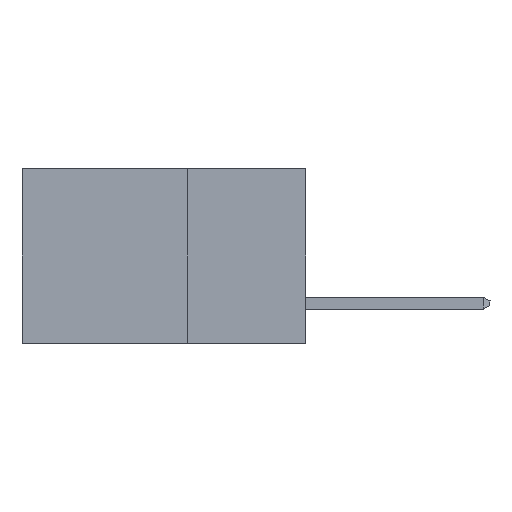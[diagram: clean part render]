
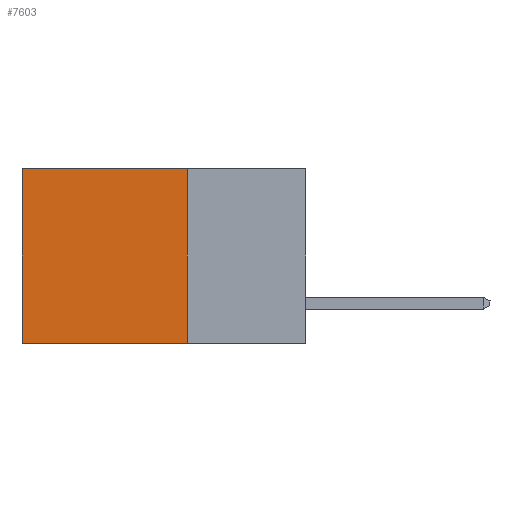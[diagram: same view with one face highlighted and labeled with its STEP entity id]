
A CAD part, left-side view. The second image highlights one B-rep face of the part: STEP entity #7603.
In plain terms, the highlighted planar face has unit normal (-1, 0, 0).
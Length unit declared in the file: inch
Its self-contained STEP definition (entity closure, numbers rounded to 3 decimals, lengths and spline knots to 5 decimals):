
#1020 = VERTEX_POINT ( 'NONE', #2128 ) ;
#2128 = CARTESIAN_POINT ( 'NONE',  ( 0.298, 0.25, -0.37 ) ) ;
#2580 = EDGE_LOOP ( 'NONE', ( #7475, #16033, #7656, #6407 ) ) ;
#3238 = LINE ( 'NONE', #11141, #9795 ) ;
#3564 = DIRECTION ( 'NONE',  ( 0., 1., 0. ) ) ;
#3631 = LINE ( 'NONE', #15164, #6286 ) ;
#3902 = AXIS2_PLACEMENT_3D ( 'NONE', #6170, #16799, #8783 ) ;
#5137 = VECTOR ( 'NONE', #12179, 39.37008 ) ;
#5731 = EDGE_CURVE ( 'NONE', #11971, #14548, #3631, .T. ) ;
#6170 = CARTESIAN_POINT ( 'NONE',  ( 0.298, 0.25, 0. ) ) ;
#6286 = VECTOR ( 'NONE', #11231, 39.37008 ) ;
#6407 = ORIENTED_EDGE ( 'NONE', *, *, #7069, .T. ) ;
#7069 = EDGE_CURVE ( 'NONE', #8485, #11971, #15733, .T. ) ;
#7475 = ORIENTED_EDGE ( 'NONE', *, *, #5731, .T. ) ;
#7603 = ADVANCED_FACE ( 'NONE', ( #16939 ), #15314, .F. ) ;
#7610 = CARTESIAN_POINT ( 'NONE',  ( 0.298, 0.6, -0.37 ) ) ;
#7656 = ORIENTED_EDGE ( 'NONE', *, *, #8332, .F. ) ;
#8162 = CARTESIAN_POINT ( 'NONE',  ( 0.298, 0.6, 0. ) ) ;
#8332 = EDGE_CURVE ( 'NONE', #8485, #1020, #3238, .T. ) ;
#8485 = VERTEX_POINT ( 'NONE', #12926 ) ;
#8783 = DIRECTION ( 'NONE',  ( 0., 0., -1. ) ) ;
#9545 = VECTOR ( 'NONE', #3564, 39.37008 ) ;
#9795 = VECTOR ( 'NONE', #13102, 39.37008 ) ;
#11141 = CARTESIAN_POINT ( 'NONE',  ( 0.298, 0.25, 0. ) ) ;
#11221 = CARTESIAN_POINT ( 'NONE',  ( 0.298, 0.25, -0.37 ) ) ;
#11231 = DIRECTION ( 'NONE',  ( 0., 0., -1. ) ) ;
#11971 = VERTEX_POINT ( 'NONE', #8162 ) ;
#12179 = DIRECTION ( 'NONE',  ( 0., 1., 0. ) ) ;
#12318 = EDGE_CURVE ( 'NONE', #1020, #14548, #12521, .T. ) ;
#12521 = LINE ( 'NONE', #11221, #9545 ) ;
#12926 = CARTESIAN_POINT ( 'NONE',  ( 0.298, 0.25, 0. ) ) ;
#13102 = DIRECTION ( 'NONE',  ( 0., 0., -1. ) ) ;
#13706 = CARTESIAN_POINT ( 'NONE',  ( 0.298, 0.25, 0. ) ) ;
#14548 = VERTEX_POINT ( 'NONE', #7610 ) ;
#15164 = CARTESIAN_POINT ( 'NONE',  ( 0.298, 0.6, 0. ) ) ;
#15314 = PLANE ( 'NONE',  #3902 ) ;
#15733 = LINE ( 'NONE', #13706, #5137 ) ;
#16033 = ORIENTED_EDGE ( 'NONE', *, *, #12318, .F. ) ;
#16799 = DIRECTION ( 'NONE',  ( 1., 0., 0. ) ) ;
#16939 = FACE_OUTER_BOUND ( 'NONE', #2580, .T. ) ;
